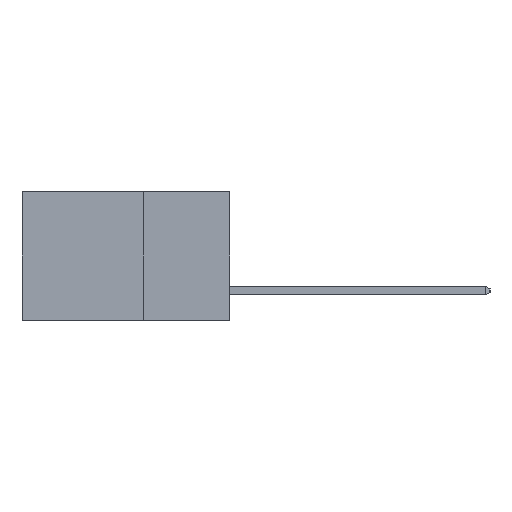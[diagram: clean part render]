
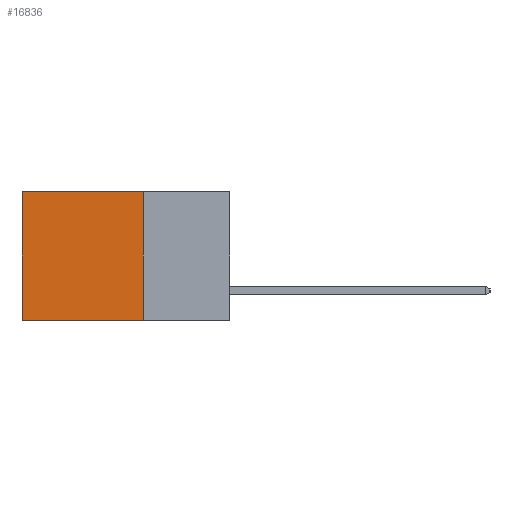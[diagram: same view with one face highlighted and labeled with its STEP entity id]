
A CAD part, left-side view. The second image highlights one B-rep face of the part: STEP entity #16836.
In plain terms, the highlighted planar face has unit normal (-1, 0, 0).
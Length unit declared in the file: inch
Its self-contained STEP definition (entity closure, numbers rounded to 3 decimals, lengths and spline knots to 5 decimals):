
#91 = VERTEX_POINT ( 'NONE', #9668 ) ;
#954 = CARTESIAN_POINT ( 'NONE',  ( 0.298, 0.25, 0. ) ) ;
#1475 = DIRECTION ( 'NONE',  ( 0., 1., 0. ) ) ;
#1831 = DIRECTION ( 'NONE',  ( 0., 0., -1. ) ) ;
#1971 = VERTEX_POINT ( 'NONE', #18157 ) ;
#2141 = FACE_OUTER_BOUND ( 'NONE', #4989, .T. ) ;
#2252 = VECTOR ( 'NONE', #17157, 39.37008 ) ;
#2708 = EDGE_CURVE ( 'NONE', #8609, #19669, #14756, .T. ) ;
#4215 = EDGE_CURVE ( 'NONE', #8609, #91, #13109, .T. ) ;
#4430 = DIRECTION ( 'NONE',  ( 0., 0., -1. ) ) ;
#4989 = EDGE_LOOP ( 'NONE', ( #13194, #9803, #11627, #19241 ) ) ;
#5587 = VECTOR ( 'NONE', #8558, 39.37008 ) ;
#6316 = CARTESIAN_POINT ( 'NONE',  ( 0.298, 0.25, 0. ) ) ;
#8275 = LINE ( 'NONE', #21809, #16739 ) ;
#8558 = DIRECTION ( 'NONE',  ( 0., 0., -1. ) ) ;
#8609 = VERTEX_POINT ( 'NONE', #954 ) ;
#9668 = CARTESIAN_POINT ( 'NONE',  ( 0.298, 0.6, 0. ) ) ;
#9803 = ORIENTED_EDGE ( 'NONE', *, *, #14284, .F. ) ;
#10527 = PLANE ( 'NONE',  #16323 ) ;
#11140 = CARTESIAN_POINT ( 'NONE',  ( 0.298, 0.25, -0.37 ) ) ;
#11627 = ORIENTED_EDGE ( 'NONE', *, *, #2708, .F. ) ;
#12263 = DIRECTION ( 'NONE',  ( 1., 0., 0. ) ) ;
#13109 = LINE ( 'NONE', #6316, #2252 ) ;
#13194 = ORIENTED_EDGE ( 'NONE', *, *, #18760, .T. ) ;
#14284 = EDGE_CURVE ( 'NONE', #19669, #1971, #8275, .T. ) ;
#14756 = LINE ( 'NONE', #15438, #19161 ) ;
#15438 = CARTESIAN_POINT ( 'NONE',  ( 0.298, 0.25, 0. ) ) ;
#16323 = AXIS2_PLACEMENT_3D ( 'NONE', #17208, #12263, #1831 ) ;
#16739 = VECTOR ( 'NONE', #1475, 39.37008 ) ;
#16836 = ADVANCED_FACE ( 'NONE', ( #2141 ), #10527, .F. ) ;
#17157 = DIRECTION ( 'NONE',  ( 0., 1., 0. ) ) ;
#17208 = CARTESIAN_POINT ( 'NONE',  ( 0.298, 0.25, 0. ) ) ;
#18157 = CARTESIAN_POINT ( 'NONE',  ( 0.298, 0.6, -0.37 ) ) ;
#18600 = LINE ( 'NONE', #18650, #5587 ) ;
#18650 = CARTESIAN_POINT ( 'NONE',  ( 0.298, 0.6, 0. ) ) ;
#18760 = EDGE_CURVE ( 'NONE', #91, #1971, #18600, .T. ) ;
#19161 = VECTOR ( 'NONE', #4430, 39.37008 ) ;
#19241 = ORIENTED_EDGE ( 'NONE', *, *, #4215, .T. ) ;
#19669 = VERTEX_POINT ( 'NONE', #11140 ) ;
#21809 = CARTESIAN_POINT ( 'NONE',  ( 0.298, 0.25, -0.37 ) ) ;
